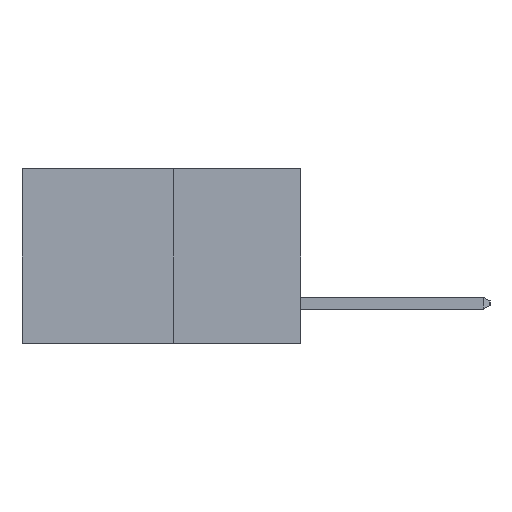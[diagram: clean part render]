
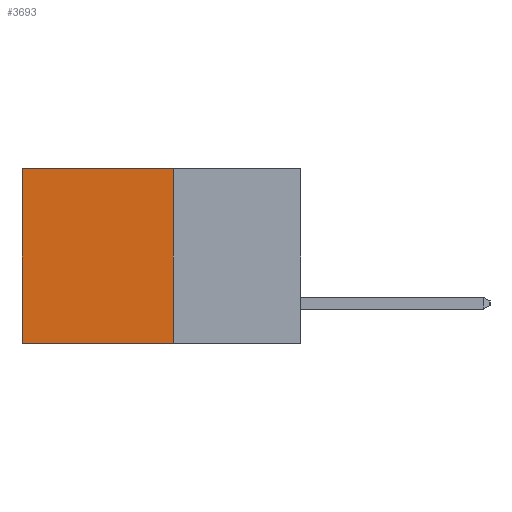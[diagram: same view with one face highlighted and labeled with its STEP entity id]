
A CAD part, left-side view. The second image highlights one B-rep face of the part: STEP entity #3693.
In plain terms, the highlighted planar face has unit normal (-1, 0, 0).
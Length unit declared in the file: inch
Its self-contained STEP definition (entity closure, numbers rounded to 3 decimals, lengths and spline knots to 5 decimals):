
#56 = PLANE ( 'NONE',  #1386 ) ;
#110 = LINE ( 'NONE', #1151, #8169 ) ;
#565 = ORIENTED_EDGE ( 'NONE', *, *, #7361, .T. ) ;
#881 = ORIENTED_EDGE ( 'NONE', *, *, #2917, .F. ) ;
#921 = ORIENTED_EDGE ( 'NONE', *, *, #6201, .T. ) ;
#1151 = CARTESIAN_POINT ( 'NONE',  ( 0.277, 0.59, -0.37 ) ) ;
#1181 = VECTOR ( 'NONE', #1427, 39.37008 ) ;
#1386 = AXIS2_PLACEMENT_3D ( 'NONE', #2415, #3510, #5132 ) ;
#1427 = DIRECTION ( 'NONE',  ( 0., 1., 0. ) ) ;
#1565 = FACE_OUTER_BOUND ( 'NONE', #3078, .T. ) ;
#1570 = VECTOR ( 'NONE', #5894, 39.37008 ) ;
#2064 = CARTESIAN_POINT ( 'NONE',  ( 0.277, 0.27, -0.37 ) ) ;
#2415 = CARTESIAN_POINT ( 'NONE',  ( 0.277, 0.27, -0.37 ) ) ;
#2857 = CARTESIAN_POINT ( 'NONE',  ( 0.277, 0.27, -0.37 ) ) ;
#2900 = LINE ( 'NONE', #5903, #1181 ) ;
#2917 = EDGE_CURVE ( 'NONE', #6090, #5707, #2900, .T. ) ;
#3078 = EDGE_LOOP ( 'NONE', ( #565, #881, #5207, #921 ) ) ;
#3273 = VERTEX_POINT ( 'NONE', #8027 ) ;
#3510 = DIRECTION ( 'NONE',  ( 1., 0., 0. ) ) ;
#3693 = ADVANCED_FACE ( 'NONE', ( #1565 ), #56, .F. ) ;
#4352 = EDGE_CURVE ( 'NONE', #3273, #6090, #7782, .T. ) ;
#5132 = DIRECTION ( 'NONE',  ( 0., 0., -1. ) ) ;
#5207 = ORIENTED_EDGE ( 'NONE', *, *, #4352, .F. ) ;
#5707 = VERTEX_POINT ( 'NONE', #6401 ) ;
#5774 = VERTEX_POINT ( 'NONE', #6863 ) ;
#5894 = DIRECTION ( 'NONE',  ( 0., 1., 0. ) ) ;
#5903 = CARTESIAN_POINT ( 'NONE',  ( 0.277, 0.27, -0.37 ) ) ;
#6090 = VERTEX_POINT ( 'NONE', #2857 ) ;
#6116 = VECTOR ( 'NONE', #6325, 39.37008 ) ;
#6201 = EDGE_CURVE ( 'NONE', #3273, #5774, #6429, .T. ) ;
#6325 = DIRECTION ( 'NONE',  ( 0., 0., -1. ) ) ;
#6401 = CARTESIAN_POINT ( 'NONE',  ( 0.277, 0.59, -0.37 ) ) ;
#6429 = LINE ( 'NONE', #7624, #1570 ) ;
#6863 = CARTESIAN_POINT ( 'NONE',  ( 0.277, 0.59, 0. ) ) ;
#7361 = EDGE_CURVE ( 'NONE', #5774, #5707, #110, .T. ) ;
#7497 = DIRECTION ( 'NONE',  ( 0., 0., -1. ) ) ;
#7624 = CARTESIAN_POINT ( 'NONE',  ( 0.277, 0.27, 0. ) ) ;
#7782 = LINE ( 'NONE', #2064, #6116 ) ;
#8027 = CARTESIAN_POINT ( 'NONE',  ( 0.277, 0.27, 0. ) ) ;
#8169 = VECTOR ( 'NONE', #7497, 39.37008 ) ;
